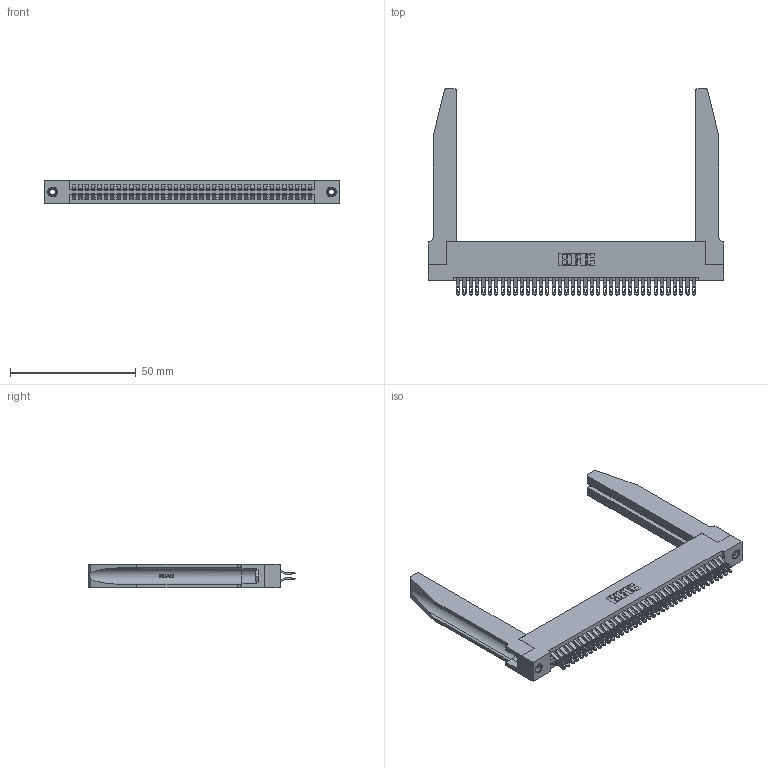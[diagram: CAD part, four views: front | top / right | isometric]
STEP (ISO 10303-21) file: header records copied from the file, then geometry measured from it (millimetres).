
FILE_DESCRIPTION (( 'STEP AP203' ), '1' );
FILE_NAME ('345-076-555-278.STEP', '2019-10-31T13:18:59', ( '' ), ( '' ), 'SwSTEP 2.0', 'SolidWorks 2016', '' );
FILE_SCHEMA (( 'CONFIG_CONTROL_DESIGN' ));
Length unit declared in the file: inch
Products named in the file (5): 345-220-078_345-220-078; 345-076-555-278; 345-250-001_345-250-001-102; 345-292-001_555 Tail; 345 Part_Flush Mounting Lugs - 0.156 Dia-TH
Assembly tree (81 placements, depth 2):
  345-076-555-278
    345 Part_Flush Mounting Lugs - 0.156 Dia-TH
    345-292-001_555 Tail  x76
    345-250-001_345-250-001-102  x2
    345-220-078_345-220-078  x2
Bounding box: 117.75 x 82.09 x 9.4 mm (x, y, z)
Volume: 19392.5 mm3; surface area: 24707.1 mm2
Topology: 81 solids, 81 shells, 4616 faces, 14401 edges, 9590 vertices
Faces by surface type: plane 2578, cylinder 1986, bspline 36, cone 12, torus 4
Entity records: 35420 total; most frequent: CARTESIAN_POINT 6893, ORIENTED_EDGE 5694, DIRECTION 5045, EDGE_CURVE 2847, LINE 2449, VECTOR 2449, VERTEX_POINT 1892, AXIS2_PLACEMENT_3D 1298
